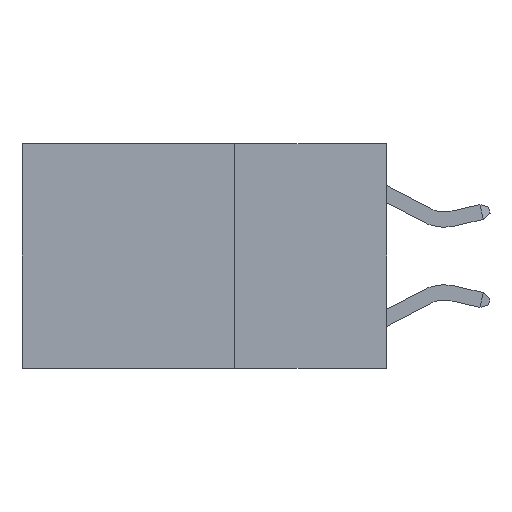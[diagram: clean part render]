
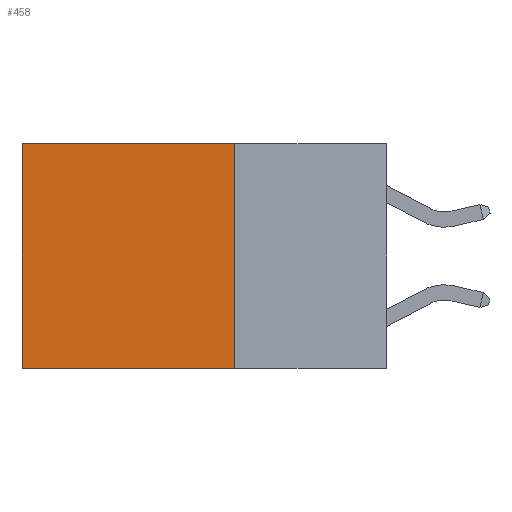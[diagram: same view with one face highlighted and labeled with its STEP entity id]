
A CAD part, left-side view. The second image highlights one B-rep face of the part: STEP entity #458.
In plain terms, the highlighted planar face has unit normal (-1, 0, 0).
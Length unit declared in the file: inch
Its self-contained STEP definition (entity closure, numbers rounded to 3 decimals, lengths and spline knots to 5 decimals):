
#155 = ORIENTED_EDGE ( 'NONE', *, *, #7161, .T. ) ;
#244 = EDGE_CURVE ( 'NONE', #9742, #5709, #3611, .T. ) ;
#404 = LINE ( 'NONE', #15341, #12260 ) ;
#458 = ADVANCED_FACE ( 'NONE', ( #13895 ), #12710, .F. ) ;
#778 = EDGE_CURVE ( 'NONE', #9742, #14639, #404, .T. ) ;
#1137 = DIRECTION ( 'NONE',  ( 0., 1., 0. ) ) ;
#1177 = EDGE_CURVE ( 'NONE', #5709, #11971, #10783, .T. ) ;
#1420 = CARTESIAN_POINT ( 'NONE',  ( 0.2625, 0.6, 0. ) ) ;
#3320 = CARTESIAN_POINT ( 'NONE',  ( 0.2625, 0.25, -0.37 ) ) ;
#3364 = VECTOR ( 'NONE', #6071, 39.37008 ) ;
#3407 = CARTESIAN_POINT ( 'NONE',  ( 0.2625, 0.25, 0. ) ) ;
#3611 = LINE ( 'NONE', #3407, #9697 ) ;
#3658 = CARTESIAN_POINT ( 'NONE',  ( 0.2625, 0.25, -0.37 ) ) ;
#3806 = DIRECTION ( 'NONE',  ( 0., 0., -1. ) ) ;
#3939 = CARTESIAN_POINT ( 'NONE',  ( 0.2625, 0.25, 0. ) ) ;
#4097 = CARTESIAN_POINT ( 'NONE',  ( 0.2625, 0.6, -0.37 ) ) ;
#4339 = VECTOR ( 'NONE', #3806, 39.37008 ) ;
#4408 = ORIENTED_EDGE ( 'NONE', *, *, #778, .T. ) ;
#5709 = VERTEX_POINT ( 'NONE', #3320 ) ;
#5916 = CARTESIAN_POINT ( 'NONE',  ( 0.2625, 0.6, 0. ) ) ;
#6071 = DIRECTION ( 'NONE',  ( 0., 1., 0. ) ) ;
#7161 = EDGE_CURVE ( 'NONE', #14639, #11971, #9325, .T. ) ;
#8313 = AXIS2_PLACEMENT_3D ( 'NONE', #15109, #10421, #13936 ) ;
#9325 = LINE ( 'NONE', #5916, #4339 ) ;
#9697 = VECTOR ( 'NONE', #12728, 39.37008 ) ;
#9742 = VERTEX_POINT ( 'NONE', #3939 ) ;
#10421 = DIRECTION ( 'NONE',  ( 1., 0., 0. ) ) ;
#10783 = LINE ( 'NONE', #3658, #3364 ) ;
#11971 = VERTEX_POINT ( 'NONE', #4097 ) ;
#12260 = VECTOR ( 'NONE', #1137, 39.37008 ) ;
#12710 = PLANE ( 'NONE',  #8313 ) ;
#12728 = DIRECTION ( 'NONE',  ( 0., 0., -1. ) ) ;
#13796 = ORIENTED_EDGE ( 'NONE', *, *, #1177, .F. ) ;
#13895 = FACE_OUTER_BOUND ( 'NONE', #14546, .T. ) ;
#13936 = DIRECTION ( 'NONE',  ( 0., 0., -1. ) ) ;
#14546 = EDGE_LOOP ( 'NONE', ( #155, #13796, #14788, #4408 ) ) ;
#14639 = VERTEX_POINT ( 'NONE', #1420 ) ;
#14788 = ORIENTED_EDGE ( 'NONE', *, *, #244, .F. ) ;
#15109 = CARTESIAN_POINT ( 'NONE',  ( 0.2625, 0.25, 0. ) ) ;
#15341 = CARTESIAN_POINT ( 'NONE',  ( 0.2625, 0.25, 0. ) ) ;
